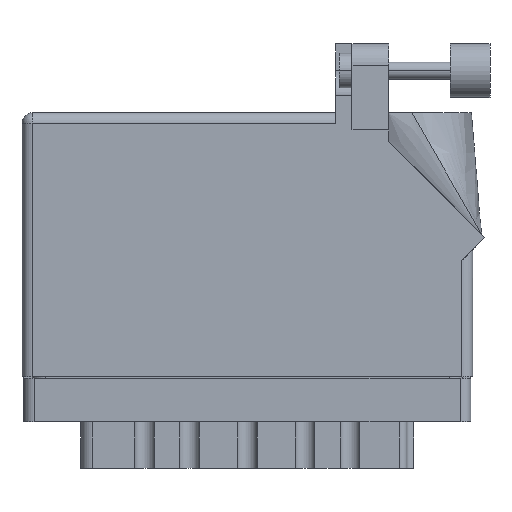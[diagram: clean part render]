
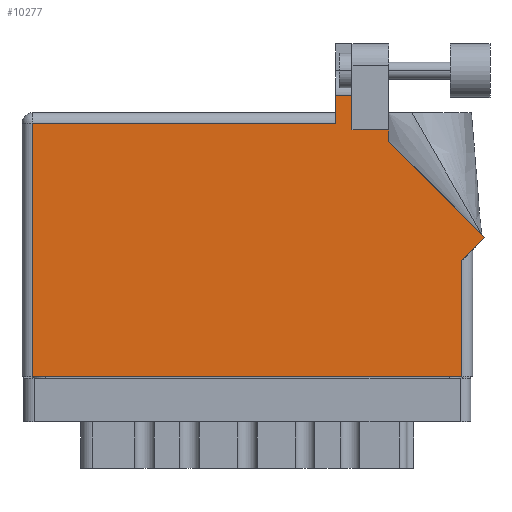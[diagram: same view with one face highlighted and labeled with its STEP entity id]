
A CAD part, front view. The second image highlights one B-rep face of the part: STEP entity #10277.
In plain terms, the highlighted face is planar.
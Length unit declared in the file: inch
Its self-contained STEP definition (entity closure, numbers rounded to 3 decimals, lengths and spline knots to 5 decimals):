
#224 = ORIENTED_EDGE ( 'NONE', *, *, #16296, .T. ) ;
#270 = EDGE_CURVE ( 'NONE', #8457, #30991, #29017, .T. ) ;
#489 = CARTESIAN_POINT ( 'NONE',  ( 1.913, 1.43, 0. ) ) ;
#642 = CARTESIAN_POINT ( 'NONE',  ( 2.126, 1.36442, 0. ) ) ;
#1312 = VECTOR ( 'NONE', #26427, 39.37008 ) ;
#1453 = VECTOR ( 'NONE', #47182, 39.37008 ) ;
#1942 = VECTOR ( 'NONE', #24942, 39.37008 ) ;
#2231 = VECTOR ( 'NONE', #12063, 39.37008 ) ;
#2808 = ORIENTED_EDGE ( 'NONE', *, *, #13475, .T. ) ;
#2855 = ORIENTED_EDGE ( 'NONE', *, *, #15749, .T. ) ;
#3020 = VECTOR ( 'NONE', #20568, 39.37008 ) ;
#3494 = VERTEX_POINT ( 'NONE', #17761 ) ;
#3511 = LINE ( 'NONE', #34759, #34285 ) ;
#4264 = VECTOR ( 'NONE', #26047, 39.37008 ) ;
#4286 = CARTESIAN_POINT ( 'NONE',  ( 2.68271, 0.80771, 0. ) ) ;
#4808 = AXIS2_PLACEMENT_3D ( 'NONE', #12438, #36150, #8858 ) ;
#4953 = EDGE_CURVE ( 'NONE', #9190, #3494, #26157, .T. ) ;
#5411 = LINE ( 'NONE', #43094, #3020 ) ;
#6423 = VERTEX_POINT ( 'NONE', #642 ) ;
#6646 = ORIENTED_EDGE ( 'NONE', *, *, #20388, .T. ) ;
#6996 = CARTESIAN_POINT ( 'NONE',  ( 2.55, 0.737, 0. ) ) ;
#7881 = DIRECTION ( 'NONE',  ( -1., 0., 0. ) ) ;
#8457 = VERTEX_POINT ( 'NONE', #14261 ) ;
#8858 = DIRECTION ( 'NONE',  ( -1., 0., 0. ) ) ;
#9190 = VERTEX_POINT ( 'NONE', #45279 ) ;
#10046 = LINE ( 'NONE', #44309, #25106 ) ;
#10277 = ADVANCED_FACE ( 'NONE', ( #44551 ), #27908, .F. ) ;
#10348 = LINE ( 'NONE', #33393, #32036 ) ;
#11551 = VERTEX_POINT ( 'NONE', #23587 ) ;
#12063 = DIRECTION ( 'NONE',  ( -1., 0., 0. ) ) ;
#12438 = CARTESIAN_POINT ( 'NONE',  ( 0., 1.53, 0. ) ) ;
#13420 = LINE ( 'NONE', #16513, #1942 ) ;
#13475 = EDGE_CURVE ( 'NONE', #39140, #9190, #17916, .T. ) ;
#13966 = LINE ( 'NONE', #42559, #35632 ) ;
#14261 = CARTESIAN_POINT ( 'NONE',  ( 2.55, 0., 0. ) ) ;
#15663 = ORIENTED_EDGE ( 'NONE', *, *, #16103, .T. ) ;
#15718 = CARTESIAN_POINT ( 'NONE',  ( 1.819, 1.468, 0. ) ) ;
#15749 = EDGE_CURVE ( 'NONE', #3494, #8457, #13420, .T. ) ;
#16103 = EDGE_CURVE ( 'NONE', #42594, #6423, #44719, .T. ) ;
#16233 = CARTESIAN_POINT ( 'NONE',  ( 0.062, 0., 0. ) ) ;
#16296 = EDGE_CURVE ( 'NONE', #47004, #24172, #13966, .T. ) ;
#16513 = CARTESIAN_POINT ( 'NONE',  ( 0., 0., 0. ) ) ;
#17761 = CARTESIAN_POINT ( 'NONE',  ( 0.062, 0., 0. ) ) ;
#17916 = LINE ( 'NONE', #43013, #2231 ) ;
#18877 = CARTESIAN_POINT ( 'NONE',  ( 2.126, 1.43, 0. ) ) ;
#20103 = CARTESIAN_POINT ( 'NONE',  ( 1.913, 1.6315, 0. ) ) ;
#20388 = EDGE_CURVE ( 'NONE', #30991, #42594, #3511, .T. ) ;
#20568 = DIRECTION ( 'NONE',  ( 0., 1., 0. ) ) ;
#20853 = ORIENTED_EDGE ( 'NONE', *, *, #48573, .T. ) ;
#22434 = DIRECTION ( 'NONE',  ( 0., -1., 0. ) ) ;
#23052 = EDGE_LOOP ( 'NONE', ( #42101, #49354, #20853, #2808, #48530, #2855, #44331, #6646, #15663, #34478, #224 ) ) ;
#23587 = CARTESIAN_POINT ( 'NONE',  ( 1.819, 1.6315, 0. ) ) ;
#24172 = VERTEX_POINT ( 'NONE', #489 ) ;
#24942 = DIRECTION ( 'NONE',  ( 1., 0., 0. ) ) ;
#25106 = VECTOR ( 'NONE', #36742, 39.37008 ) ;
#25994 = VECTOR ( 'NONE', #22434, 39.37008 ) ;
#26047 = DIRECTION ( 'NONE',  ( 0., 1., 0. ) ) ;
#26157 = LINE ( 'NONE', #16233, #1453 ) ;
#26427 = DIRECTION ( 'NONE',  ( -0.707, 0.707, 0. ) ) ;
#27908 = PLANE ( 'NONE',  #4808 ) ;
#29017 = LINE ( 'NONE', #6996, #4264 ) ;
#30016 = DIRECTION ( 'NONE',  ( 0., 1., 0. ) ) ;
#30991 = VERTEX_POINT ( 'NONE', #34664 ) ;
#32036 = VECTOR ( 'NONE', #30016, 39.37008 ) ;
#33393 = CARTESIAN_POINT ( 'NONE',  ( 2.126, 1.36442, 0. ) ) ;
#34285 = VECTOR ( 'NONE', #39080, 39.37008 ) ;
#34478 = ORIENTED_EDGE ( 'NONE', *, *, #48547, .T. ) ;
#34664 = CARTESIAN_POINT ( 'NONE',  ( 2.55, 0.675, 0. ) ) ;
#34759 = CARTESIAN_POINT ( 'NONE',  ( 2.612, 0.737, 0. ) ) ;
#34997 = VERTEX_POINT ( 'NONE', #20103 ) ;
#35632 = VECTOR ( 'NONE', #7881, 39.37008 ) ;
#36150 = DIRECTION ( 'NONE',  ( 0., 0., -1. ) ) ;
#36742 = DIRECTION ( 'NONE',  ( -1., 0., 0. ) ) ;
#36847 = EDGE_CURVE ( 'NONE', #24172, #34997, #5411, .T. ) ;
#38624 = LINE ( 'NONE', #41425, #25994 ) ;
#39080 = DIRECTION ( 'NONE',  ( 0.707, 0.707, 0. ) ) ;
#39140 = VERTEX_POINT ( 'NONE', #15718 ) ;
#41425 = CARTESIAN_POINT ( 'NONE',  ( 1.819, 1.53, 0. ) ) ;
#42101 = ORIENTED_EDGE ( 'NONE', *, *, #36847, .T. ) ;
#42219 = CARTESIAN_POINT ( 'NONE',  ( 2.68271, 0.80771, 0. ) ) ;
#42559 = CARTESIAN_POINT ( 'NONE',  ( 2.126, 1.43, 0. ) ) ;
#42594 = VERTEX_POINT ( 'NONE', #4286 ) ;
#43013 = CARTESIAN_POINT ( 'NONE',  ( 0., 1.468, 0. ) ) ;
#43094 = CARTESIAN_POINT ( 'NONE',  ( 1.913, 1.43, 0. ) ) ;
#43610 = EDGE_CURVE ( 'NONE', #34997, #11551, #10046, .T. ) ;
#44309 = CARTESIAN_POINT ( 'NONE',  ( 2.24377, 1.6315, 0. ) ) ;
#44331 = ORIENTED_EDGE ( 'NONE', *, *, #270, .T. ) ;
#44551 = FACE_OUTER_BOUND ( 'NONE', #23052, .T. ) ;
#44719 = LINE ( 'NONE', #42219, #1312 ) ;
#45279 = CARTESIAN_POINT ( 'NONE',  ( 0.062, 1.468, 0. ) ) ;
#47004 = VERTEX_POINT ( 'NONE', #18877 ) ;
#47182 = DIRECTION ( 'NONE',  ( 0., -1., 0. ) ) ;
#48530 = ORIENTED_EDGE ( 'NONE', *, *, #4953, .T. ) ;
#48547 = EDGE_CURVE ( 'NONE', #6423, #47004, #10348, .T. ) ;
#48573 = EDGE_CURVE ( 'NONE', #11551, #39140, #38624, .T. ) ;
#49354 = ORIENTED_EDGE ( 'NONE', *, *, #43610, .T. ) ;
